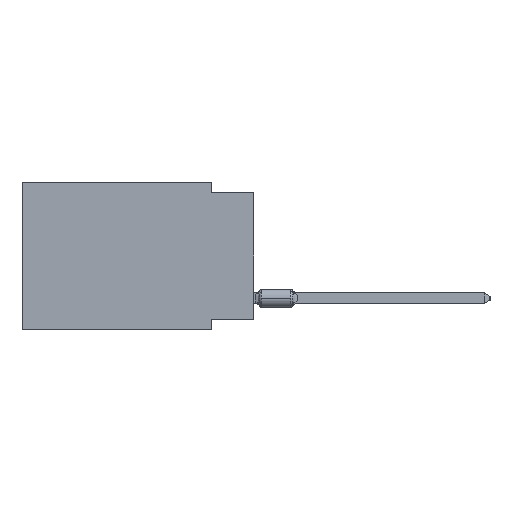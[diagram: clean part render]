
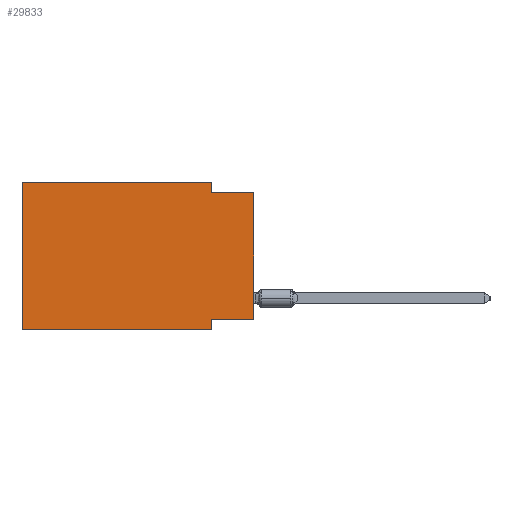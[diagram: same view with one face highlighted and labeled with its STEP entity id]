
A CAD part, left-side view. The second image highlights one B-rep face of the part: STEP entity #29833.
In plain terms, the highlighted planar face has unit normal (-1, 0, 0).
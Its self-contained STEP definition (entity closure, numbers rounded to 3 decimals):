
#5872 = LINE ( 'NONE', #64982, #22390 ) ;
#6366 = CARTESIAN_POINT ( 'NONE',  ( 0., 0., -8.255 ) ) ;
#6874 = ORIENTED_EDGE ( 'NONE', *, *, #32956, .F. ) ;
#7401 = CARTESIAN_POINT ( 'NONE',  ( 0., 13.97, 0. ) ) ;
#8094 = EDGE_CURVE ( 'NONE', #45130, #93033, #5872, .T. ) ;
#10508 = VECTOR ( 'NONE', #64788, 1000. ) ;
#10991 = ORIENTED_EDGE ( 'NONE', *, *, #76193, .F. ) ;
#13262 = LINE ( 'NONE', #71906, #81435 ) ;
#13305 = LINE ( 'NONE', #65688, #70122 ) ;
#15470 = VECTOR ( 'NONE', #15793, 1000. ) ;
#15793 = DIRECTION ( 'NONE',  ( 0., -1., 0. ) ) ;
#15806 = VERTEX_POINT ( 'NONE', #87903 ) ;
#17617 = DIRECTION ( 'NONE',  ( 1., 0., 0. ) ) ;
#18109 = PLANE ( 'NONE',  #59203 ) ;
#18550 = VERTEX_POINT ( 'NONE', #7401 ) ;
#22390 = VECTOR ( 'NONE', #79418, 1000. ) ;
#23488 = CARTESIAN_POINT ( 'NONE',  ( 0., 0., -0.635 ) ) ;
#24384 = CARTESIAN_POINT ( 'NONE',  ( 0., 13.97, 0. ) ) ;
#24828 = ORIENTED_EDGE ( 'NONE', *, *, #74691, .F. ) ;
#26836 = LINE ( 'NONE', #56171, #10508 ) ;
#27978 = ORIENTED_EDGE ( 'NONE', *, *, #72636, .F. ) ;
#28152 = DIRECTION ( 'NONE',  ( 0., -1., 0. ) ) ;
#29751 = ORIENTED_EDGE ( 'NONE', *, *, #73875, .T. ) ;
#29833 = ADVANCED_FACE ( 'NONE', ( #68119 ), #18109, .F. ) ;
#32415 = VECTOR ( 'NONE', #90259, 1000. ) ;
#32532 = ORIENTED_EDGE ( 'NONE', *, *, #8094, .F. ) ;
#32956 = EDGE_CURVE ( 'NONE', #40348, #53741, #26836, .T. ) ;
#40348 = VERTEX_POINT ( 'NONE', #53565 ) ;
#43564 = DIRECTION ( 'NONE',  ( 0., 1., 0. ) ) ;
#43594 = CARTESIAN_POINT ( 'NONE',  ( 0., 0., -0.635 ) ) ;
#45130 = VERTEX_POINT ( 'NONE', #66173 ) ;
#47212 = ORIENTED_EDGE ( 'NONE', *, *, #85562, .F. ) ;
#51564 = VERTEX_POINT ( 'NONE', #43594 ) ;
#53565 = CARTESIAN_POINT ( 'NONE',  ( 0., 2.54, 0. ) ) ;
#53725 = LINE ( 'NONE', #24384, #32415 ) ;
#53741 = VERTEX_POINT ( 'NONE', #81817 ) ;
#56171 = CARTESIAN_POINT ( 'NONE',  ( 0., 2.54, 0. ) ) ;
#59203 = AXIS2_PLACEMENT_3D ( 'NONE', #89296, #17617, #90710 ) ;
#64788 = DIRECTION ( 'NONE',  ( 0., 0., -1. ) ) ;
#64982 = CARTESIAN_POINT ( 'NONE',  ( 0., 2.54, -8.89 ) ) ;
#65688 = CARTESIAN_POINT ( 'NONE',  ( 0., 0., -8.255 ) ) ;
#66173 = CARTESIAN_POINT ( 'NONE',  ( 0., 2.54, -8.255 ) ) ;
#67820 = ORIENTED_EDGE ( 'NONE', *, *, #84648, .T. ) ;
#68119 = FACE_OUTER_BOUND ( 'NONE', #70772, .T. ) ;
#68142 = CARTESIAN_POINT ( 'NONE',  ( 0., 2.54, -8.89 ) ) ;
#70122 = VECTOR ( 'NONE', #43564, 1000. ) ;
#70772 = EDGE_LOOP ( 'NONE', ( #67820, #27978, #6874, #24828, #47212, #29751, #32532, #10991 ) ) ;
#71533 = DIRECTION ( 'NONE',  ( 0., 0., 1. ) ) ;
#71906 = CARTESIAN_POINT ( 'NONE',  ( 0., 13.97, -8.89 ) ) ;
#72636 = EDGE_CURVE ( 'NONE', #53741, #51564, #81662, .T. ) ;
#73875 = EDGE_CURVE ( 'NONE', #15806, #93033, #13262, .T. ) ;
#74691 = EDGE_CURVE ( 'NONE', #18550, #40348, #53725, .T. ) ;
#76193 = EDGE_CURVE ( 'NONE', #94326, #45130, #13305, .T. ) ;
#77200 = LINE ( 'NONE', #90210, #82760 ) ;
#79418 = DIRECTION ( 'NONE',  ( 0., 0., -1. ) ) ;
#81169 = CARTESIAN_POINT ( 'NONE',  ( 0., 0., 0. ) ) ;
#81435 = VECTOR ( 'NONE', #28152, 1000. ) ;
#81662 = LINE ( 'NONE', #23488, #15470 ) ;
#81817 = CARTESIAN_POINT ( 'NONE',  ( 0., 2.54, -0.635 ) ) ;
#82760 = VECTOR ( 'NONE', #91152, 1000. ) ;
#84648 = EDGE_CURVE ( 'NONE', #94326, #51564, #94177, .T. ) ;
#85562 = EDGE_CURVE ( 'NONE', #15806, #18550, #77200, .T. ) ;
#87903 = CARTESIAN_POINT ( 'NONE',  ( 0., 13.97, -8.89 ) ) ;
#89296 = CARTESIAN_POINT ( 'NONE',  ( 0., 13.97, 0. ) ) ;
#90210 = CARTESIAN_POINT ( 'NONE',  ( 0., 13.97, 0. ) ) ;
#90259 = DIRECTION ( 'NONE',  ( 0., -1., 0. ) ) ;
#90710 = DIRECTION ( 'NONE',  ( 0., 0., -1. ) ) ;
#91152 = DIRECTION ( 'NONE',  ( 0., 0., 1. ) ) ;
#92100 = VECTOR ( 'NONE', #71533, 1000. ) ;
#93033 = VERTEX_POINT ( 'NONE', #68142 ) ;
#94177 = LINE ( 'NONE', #81169, #92100 ) ;
#94326 = VERTEX_POINT ( 'NONE', #6366 ) ;
